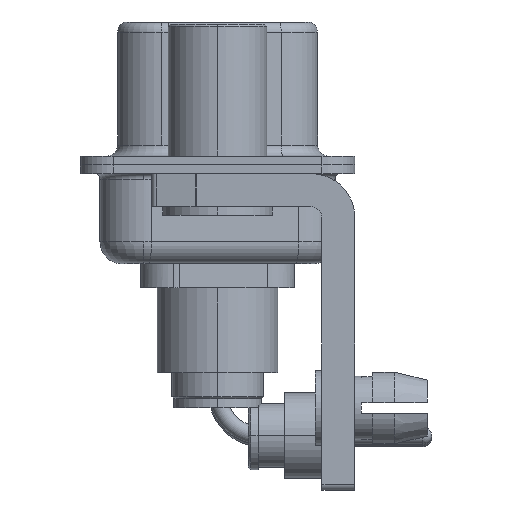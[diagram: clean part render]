
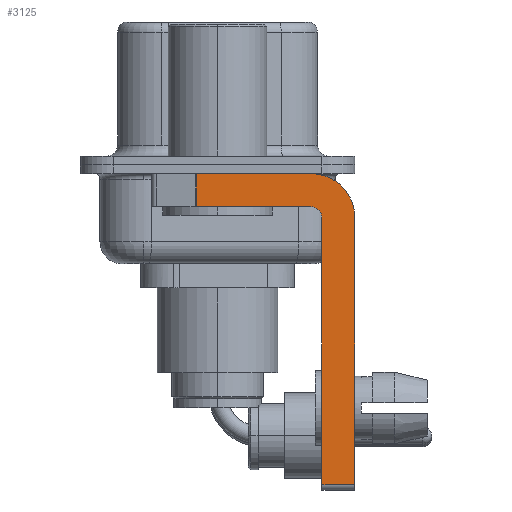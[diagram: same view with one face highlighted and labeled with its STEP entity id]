
A CAD part, left-side view. The second image highlights one B-rep face of the part: STEP entity #3125.
In plain terms, the highlighted planar face has unit normal (-1, 0, 0).
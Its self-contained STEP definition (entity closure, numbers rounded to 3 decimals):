
#37 = EDGE_CURVE ( 'NONE', #6355, #11653, #3085, .T. ) ;
#125 = CARTESIAN_POINT ( 'NONE',  ( -2.9, -4.25, -14.55 ) ) ;
#617 = PLANE ( 'NONE',  #9365 ) ;
#1020 = CARTESIAN_POINT ( 'NONE',  ( -2.9, -6.25, -2.4 ) ) ;
#1225 = ORIENTED_EDGE ( 'NONE', *, *, #10693, .F. ) ;
#1819 = LINE ( 'NONE', #125, #7915 ) ;
#1878 = CARTESIAN_POINT ( 'NONE',  ( -2.9, -4.75, -14.55 ) ) ;
#2475 = CIRCLE ( 'NONE', #12565, 0.5 ) ;
#2831 = DIRECTION ( 'NONE',  ( 0., 0., -1. ) ) ;
#3085 = LINE ( 'NONE', #6857, #16598 ) ;
#3125 = ADVANCED_FACE ( 'NONE', ( #13760 ), #617, .F. ) ;
#3180 = DIRECTION ( 'NONE',  ( 0., 0., 1. ) ) ;
#3192 = CARTESIAN_POINT ( 'NONE',  ( -2.9, -6.25, -2.4 ) ) ;
#3465 = DIRECTION ( 'NONE',  ( 0., 1., 0. ) ) ;
#5131 = EDGE_CURVE ( 'NONE', #11653, #15803, #6615, .T. ) ;
#5630 = ORIENTED_EDGE ( 'NONE', *, *, #5131, .F. ) ;
#5943 = EDGE_LOOP ( 'NONE', ( #23950, #18586, #14623, #19821, #1225, #10779, #6566, #5630 ) ) ;
#6091 = DIRECTION ( 'NONE',  ( 1., 0., 0. ) ) ;
#6355 = VERTEX_POINT ( 'NONE', #21767 ) ;
#6364 = LINE ( 'NONE', #3192, #6728 ) ;
#6566 = ORIENTED_EDGE ( 'NONE', *, *, #8056, .F. ) ;
#6615 = CIRCLE ( 'NONE', #12822, 2. ) ;
#6728 = VECTOR ( 'NONE', #2831, 1000. ) ;
#6857 = CARTESIAN_POINT ( 'NONE',  ( -2.9, 3., -0.4 ) ) ;
#7915 = VECTOR ( 'NONE', #22146, 1000. ) ;
#8056 = EDGE_CURVE ( 'NONE', #15803, #13786, #6364, .T. ) ;
#8784 = CARTESIAN_POINT ( 'NONE',  ( -2.9, -4.25, -2.4 ) ) ;
#9028 = LINE ( 'NONE', #23843, #16644 ) ;
#9365 = AXIS2_PLACEMENT_3D ( 'NONE', #17182, #6091, #18989 ) ;
#10693 = EDGE_CURVE ( 'NONE', #14082, #19672, #16450, .T. ) ;
#10734 = DIRECTION ( 'NONE',  ( 1., 0., 0. ) ) ;
#10779 = ORIENTED_EDGE ( 'NONE', *, *, #20829, .T. ) ;
#11653 = VERTEX_POINT ( 'NONE', #16280 ) ;
#12565 = AXIS2_PLACEMENT_3D ( 'NONE', #20440, #12893, #13267 ) ;
#12568 = DIRECTION ( 'NONE',  ( 0., -1., 0. ) ) ;
#12704 = LINE ( 'NONE', #20128, #14384 ) ;
#12822 = AXIS2_PLACEMENT_3D ( 'NONE', #8784, #10734, #18165 ) ;
#12893 = DIRECTION ( 'NONE',  ( -1., 0., 0. ) ) ;
#13267 = DIRECTION ( 'NONE',  ( 0., 0., 1. ) ) ;
#13314 = CARTESIAN_POINT ( 'NONE',  ( -2.9, -4.25, -1.9 ) ) ;
#13760 = FACE_OUTER_BOUND ( 'NONE', #5943, .T. ) ;
#13786 = VERTEX_POINT ( 'NONE', #20761 ) ;
#14082 = VERTEX_POINT ( 'NONE', #1878 ) ;
#14384 = VECTOR ( 'NONE', #3465, 1000. ) ;
#14585 = EDGE_CURVE ( 'NONE', #6355, #15048, #9028, .T. ) ;
#14623 = ORIENTED_EDGE ( 'NONE', *, *, #18281, .F. ) ;
#15048 = VERTEX_POINT ( 'NONE', #19957 ) ;
#15803 = VERTEX_POINT ( 'NONE', #1020 ) ;
#16280 = CARTESIAN_POINT ( 'NONE',  ( -2.9, -4.25, -0.4 ) ) ;
#16450 = LINE ( 'NONE', #18267, #16504 ) ;
#16504 = VECTOR ( 'NONE', #3180, 1000. ) ;
#16598 = VECTOR ( 'NONE', #12568, 1000. ) ;
#16644 = VECTOR ( 'NONE', #18395, 1000. ) ;
#17182 = CARTESIAN_POINT ( 'NONE',  ( -2.9, -4.25, -2.4 ) ) ;
#18165 = DIRECTION ( 'NONE',  ( 0., 0., -1. ) ) ;
#18267 = CARTESIAN_POINT ( 'NONE',  ( -2.9, -4.75, -14.8 ) ) ;
#18281 = EDGE_CURVE ( 'NONE', #18476, #15048, #12704, .T. ) ;
#18395 = DIRECTION ( 'NONE',  ( 0., 0., -1. ) ) ;
#18476 = VERTEX_POINT ( 'NONE', #13314 ) ;
#18586 = ORIENTED_EDGE ( 'NONE', *, *, #14585, .T. ) ;
#18989 = DIRECTION ( 'NONE',  ( 0., 0., -1. ) ) ;
#19672 = VERTEX_POINT ( 'NONE', #20247 ) ;
#19821 = ORIENTED_EDGE ( 'NONE', *, *, #20774, .F. ) ;
#19957 = CARTESIAN_POINT ( 'NONE',  ( -2.9, 0.978, -1.9 ) ) ;
#20128 = CARTESIAN_POINT ( 'NONE',  ( -2.9, -4.25, -1.9 ) ) ;
#20247 = CARTESIAN_POINT ( 'NONE',  ( -2.9, -4.75, -2.4 ) ) ;
#20440 = CARTESIAN_POINT ( 'NONE',  ( -2.9, -4.25, -2.4 ) ) ;
#20761 = CARTESIAN_POINT ( 'NONE',  ( -2.9, -6.25, -14.55 ) ) ;
#20774 = EDGE_CURVE ( 'NONE', #19672, #18476, #2475, .T. ) ;
#20829 = EDGE_CURVE ( 'NONE', #14082, #13786, #1819, .T. ) ;
#21767 = CARTESIAN_POINT ( 'NONE',  ( -2.9, 0.978, -0.4 ) ) ;
#22146 = DIRECTION ( 'NONE',  ( 0., -1., 0. ) ) ;
#23843 = CARTESIAN_POINT ( 'NONE',  ( -2.9, 0.978, -1.9 ) ) ;
#23950 = ORIENTED_EDGE ( 'NONE', *, *, #37, .F. ) ;
